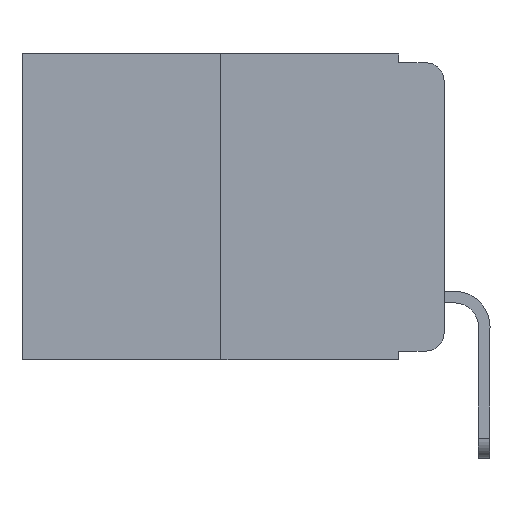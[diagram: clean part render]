
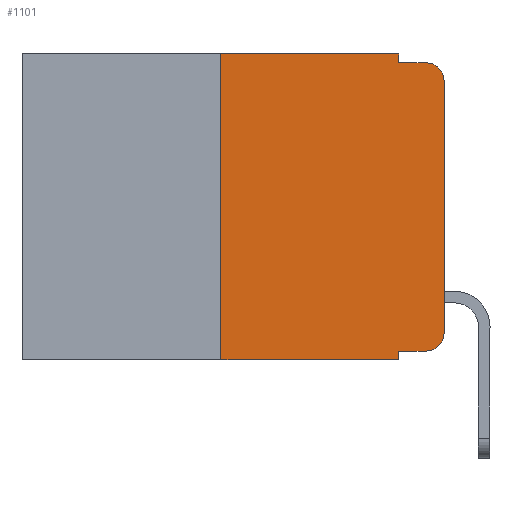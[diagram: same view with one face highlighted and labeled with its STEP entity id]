
A CAD part, left-side view. The second image highlights one B-rep face of the part: STEP entity #1101.
In plain terms, the highlighted planar face has unit normal (-1, 0, 0).
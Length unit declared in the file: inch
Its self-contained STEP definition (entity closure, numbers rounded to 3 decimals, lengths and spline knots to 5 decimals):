
#26 = ORIENTED_EDGE ( 'NONE', *, *, #6372, .T. ) ;
#230 = ORIENTED_EDGE ( 'NONE', *, *, #8920, .T. ) ;
#320 = ORIENTED_EDGE ( 'NONE', *, *, #2156, .T. ) ;
#437 = AXIS2_PLACEMENT_3D ( 'NONE', #10460, #10388, #8234 ) ;
#641 = DIRECTION ( 'NONE',  ( 0., -1., 0. ) ) ;
#758 = CARTESIAN_POINT ( 'NONE',  ( 0., 0.051, 0. ) ) ;
#768 = VERTEX_POINT ( 'NONE', #8218 ) ;
#772 = EDGE_CURVE ( 'NONE', #768, #12420, #2183, .T. ) ;
#805 = DIRECTION ( 'NONE',  ( -1., 0., 0. ) ) ;
#1050 = ORIENTED_EDGE ( 'NONE', *, *, #772, .F. ) ;
#1100 = VERTEX_POINT ( 'NONE', #11619 ) ;
#1101 = ADVANCED_FACE ( 'NONE', ( #11259 ), #11580, .F. ) ;
#1426 = CARTESIAN_POINT ( 'NONE',  ( 0., 0., 0. ) ) ;
#1502 = VECTOR ( 'NONE', #2076, 39.37008 ) ;
#1621 = VERTEX_POINT ( 'NONE', #6660 ) ;
#1633 = VECTOR ( 'NONE', #641, 39.37008 ) ;
#1726 = DIRECTION ( 'NONE',  ( 0., 0., 1. ) ) ;
#1786 = LINE ( 'NONE', #9948, #9308 ) ;
#1817 = LINE ( 'NONE', #1907, #1502 ) ;
#1907 = CARTESIAN_POINT ( 'NONE',  ( 0., 0.051, -0.333 ) ) ;
#2076 = DIRECTION ( 'NONE',  ( 0., -1., 0. ) ) ;
#2156 = EDGE_CURVE ( 'NONE', #768, #6556, #1817, .T. ) ;
#2183 = LINE ( 'NONE', #9360, #12298 ) ;
#2604 = ORIENTED_EDGE ( 'NONE', *, *, #2812, .T. ) ;
#2687 = ORIENTED_EDGE ( 'NONE', *, *, #9629, .F. ) ;
#2812 = EDGE_CURVE ( 'NONE', #6556, #5681, #9981, .T. ) ;
#3609 = EDGE_CURVE ( 'NONE', #1100, #1621, #6892, .T. ) ;
#4089 = ORIENTED_EDGE ( 'NONE', *, *, #11622, .F. ) ;
#4106 = DIRECTION ( 'NONE',  ( 0., -1., 0. ) ) ;
#4200 = ORIENTED_EDGE ( 'NONE', *, *, #12255, .F. ) ;
#4378 = VECTOR ( 'NONE', #4464, 39.37008 ) ;
#4464 = DIRECTION ( 'NONE',  ( 0., 0., 1. ) ) ;
#4571 = LINE ( 'NONE', #758, #6526 ) ;
#4970 = CARTESIAN_POINT ( 'NONE',  ( 0., 0.051, -0.343 ) ) ;
#5246 = CARTESIAN_POINT ( 'NONE',  ( 0., 0., -0.313 ) ) ;
#5531 = CARTESIAN_POINT ( 'NONE',  ( 0., 0.02, -0.01 ) ) ;
#5563 = ORIENTED_EDGE ( 'NONE', *, *, #3609, .F. ) ;
#5681 = VERTEX_POINT ( 'NONE', #5246 ) ;
#5776 = DIRECTION ( 'NONE',  ( 0., 0., -1. ) ) ;
#6372 = EDGE_CURVE ( 'NONE', #5681, #6637, #6950, .T. ) ;
#6435 = VERTEX_POINT ( 'NONE', #11397 ) ;
#6526 = VECTOR ( 'NONE', #5776, 39.37008 ) ;
#6556 = VERTEX_POINT ( 'NONE', #10609 ) ;
#6595 = VECTOR ( 'NONE', #10060, 39.37008 ) ;
#6637 = VERTEX_POINT ( 'NONE', #10750 ) ;
#6660 = CARTESIAN_POINT ( 'NONE',  ( 0., 0.051, 0. ) ) ;
#6760 = CARTESIAN_POINT ( 'NONE',  ( 0., 0.02, -0.03 ) ) ;
#6892 = LINE ( 'NONE', #11926, #1633 ) ;
#6913 = CIRCLE ( 'NONE', #10619, 0.02 ) ;
#6950 = LINE ( 'NONE', #1426, #4378 ) ;
#7000 = DIRECTION ( 'NONE',  ( 0., 0., -1. ) ) ;
#7658 = EDGE_CURVE ( 'NONE', #6637, #8499, #6913, .T. ) ;
#7743 = DIRECTION ( 'NONE',  ( 0., 0., -1. ) ) ;
#7939 = EDGE_LOOP ( 'NONE', ( #26, #8215, #2687, #4089, #5563, #4200, #230, #1050, #320, #2604 ) ) ;
#7984 = VECTOR ( 'NONE', #1726, 39.37008 ) ;
#8215 = ORIENTED_EDGE ( 'NONE', *, *, #7658, .T. ) ;
#8218 = CARTESIAN_POINT ( 'NONE',  ( 0., 0.051, -0.333 ) ) ;
#8234 = DIRECTION ( 'NONE',  ( 0., 0., -1. ) ) ;
#8499 = VERTEX_POINT ( 'NONE', #5531 ) ;
#8920 = EDGE_CURVE ( 'NONE', #6435, #12420, #11819, .T. ) ;
#9308 = VECTOR ( 'NONE', #4106, 39.37008 ) ;
#9360 = CARTESIAN_POINT ( 'NONE',  ( 0., 0.051, 0. ) ) ;
#9405 = VERTEX_POINT ( 'NONE', #12554 ) ;
#9629 = EDGE_CURVE ( 'NONE', #9405, #8499, #1786, .T. ) ;
#9948 = CARTESIAN_POINT ( 'NONE',  ( 0., 0.051, -0.01 ) ) ;
#9981 = CIRCLE ( 'NONE', #437, 0.02 ) ;
#10060 = DIRECTION ( 'NONE',  ( 0., -1., 0. ) ) ;
#10388 = DIRECTION ( 'NONE',  ( -1., 0., 0. ) ) ;
#10460 = CARTESIAN_POINT ( 'NONE',  ( 0., 0.02, -0.313 ) ) ;
#10558 = CARTESIAN_POINT ( 'NONE',  ( 0., 0.25, 0. ) ) ;
#10609 = CARTESIAN_POINT ( 'NONE',  ( 0., 0.02, -0.333 ) ) ;
#10619 = AXIS2_PLACEMENT_3D ( 'NONE', #6760, #805, #7743 ) ;
#10629 = LINE ( 'NONE', #10558, #7984 ) ;
#10750 = CARTESIAN_POINT ( 'NONE',  ( 0., 0., -0.03 ) ) ;
#11040 = AXIS2_PLACEMENT_3D ( 'NONE', #11898, #11556, #11554 ) ;
#11259 = FACE_OUTER_BOUND ( 'NONE', #7939, .T. ) ;
#11397 = CARTESIAN_POINT ( 'NONE',  ( 0., 0.25, -0.343 ) ) ;
#11554 = DIRECTION ( 'NONE',  ( 0., 0., -1. ) ) ;
#11556 = DIRECTION ( 'NONE',  ( 1., 0., 0. ) ) ;
#11580 = PLANE ( 'NONE',  #11040 ) ;
#11619 = CARTESIAN_POINT ( 'NONE',  ( 0., 0.25, 0. ) ) ;
#11622 = EDGE_CURVE ( 'NONE', #1621, #9405, #4571, .T. ) ;
#11819 = LINE ( 'NONE', #11982, #6595 ) ;
#11898 = CARTESIAN_POINT ( 'NONE',  ( 0., 0.473, 0. ) ) ;
#11926 = CARTESIAN_POINT ( 'NONE',  ( 0., 0.473, 0. ) ) ;
#11982 = CARTESIAN_POINT ( 'NONE',  ( 0., 0.473, -0.343 ) ) ;
#12255 = EDGE_CURVE ( 'NONE', #6435, #1100, #10629, .T. ) ;
#12298 = VECTOR ( 'NONE', #7000, 39.37008 ) ;
#12420 = VERTEX_POINT ( 'NONE', #4970 ) ;
#12554 = CARTESIAN_POINT ( 'NONE',  ( 0., 0.051, -0.01 ) ) ;
